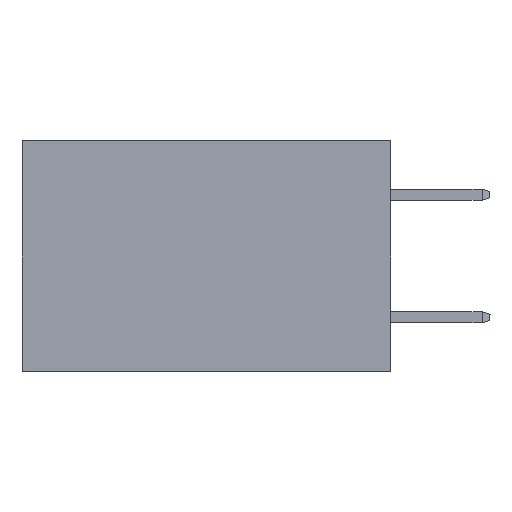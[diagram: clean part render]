
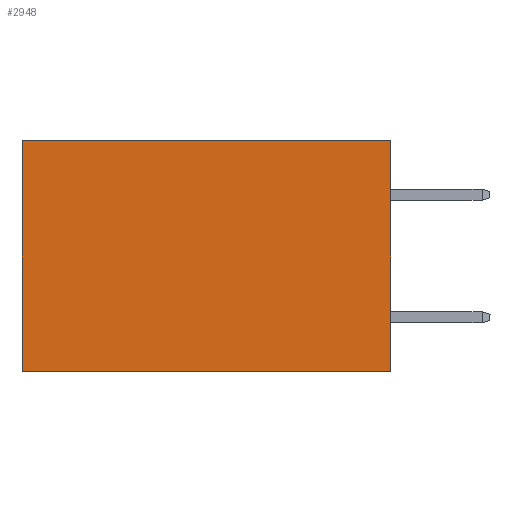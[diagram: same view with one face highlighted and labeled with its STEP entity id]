
A CAD part, left-side view. The second image highlights one B-rep face of the part: STEP entity #2948.
In plain terms, the highlighted planar face has unit normal (-1, 0, 0).
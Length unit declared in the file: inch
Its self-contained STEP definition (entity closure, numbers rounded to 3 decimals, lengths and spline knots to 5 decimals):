
#64 = VECTOR ( 'NONE', #7813, 39.37008 ) ;
#288 = EDGE_CURVE ( 'NONE', #19003, #20063, #1171, .T. ) ;
#1171 = LINE ( 'NONE', #4264, #17939 ) ;
#1609 = EDGE_CURVE ( 'NONE', #4205, #16646, #14479, .T. ) ;
#1852 = CARTESIAN_POINT ( 'NONE',  ( 0.2875, 0., -0.375 ) ) ;
#2948 = ADVANCED_FACE ( 'NONE', ( #13081 ), #15580, .F. ) ;
#3361 = LINE ( 'NONE', #10375, #5211 ) ;
#4205 = VERTEX_POINT ( 'NONE', #5260 ) ;
#4264 = CARTESIAN_POINT ( 'NONE',  ( 0.2875, 0., -0.375 ) ) ;
#5211 = VECTOR ( 'NONE', #13951, 39.37008 ) ;
#5260 = CARTESIAN_POINT ( 'NONE',  ( 0.2875, 0.6, 0. ) ) ;
#5610 = DIRECTION ( 'NONE',  ( 1., 0., 0. ) ) ;
#5905 = EDGE_LOOP ( 'NONE', ( #7347, #13079, #7869, #15262 ) ) ;
#7347 = ORIENTED_EDGE ( 'NONE', *, *, #1609, .T. ) ;
#7813 = DIRECTION ( 'NONE',  ( 0., 0., -1. ) ) ;
#7869 = ORIENTED_EDGE ( 'NONE', *, *, #288, .F. ) ;
#8055 = EDGE_CURVE ( 'NONE', #19003, #4205, #3361, .T. ) ;
#9043 = CARTESIAN_POINT ( 'NONE',  ( 0.2875, 0., -0.375 ) ) ;
#10295 = CARTESIAN_POINT ( 'NONE',  ( 0.2875, 0., -0.375 ) ) ;
#10375 = CARTESIAN_POINT ( 'NONE',  ( 0.2875, 0., 0. ) ) ;
#12633 = AXIS2_PLACEMENT_3D ( 'NONE', #9043, #5610, #15874 ) ;
#12679 = VECTOR ( 'NONE', #18633, 39.37008 ) ;
#13079 = ORIENTED_EDGE ( 'NONE', *, *, #14513, .F. ) ;
#13081 = FACE_OUTER_BOUND ( 'NONE', #5905, .T. ) ;
#13951 = DIRECTION ( 'NONE',  ( 0., 1., 0. ) ) ;
#14454 = CARTESIAN_POINT ( 'NONE',  ( 0.2875, 0.6, -0.375 ) ) ;
#14479 = LINE ( 'NONE', #14454, #64 ) ;
#14513 = EDGE_CURVE ( 'NONE', #20063, #16646, #21075, .T. ) ;
#15262 = ORIENTED_EDGE ( 'NONE', *, *, #8055, .T. ) ;
#15580 = PLANE ( 'NONE',  #12633 ) ;
#15804 = CARTESIAN_POINT ( 'NONE',  ( 0.2875, 0.6, -0.375 ) ) ;
#15874 = DIRECTION ( 'NONE',  ( 0., 0., -1. ) ) ;
#15881 = DIRECTION ( 'NONE',  ( 0., 0., -1. ) ) ;
#16646 = VERTEX_POINT ( 'NONE', #15804 ) ;
#17939 = VECTOR ( 'NONE', #15881, 39.37008 ) ;
#18633 = DIRECTION ( 'NONE',  ( 0., 1., 0. ) ) ;
#19003 = VERTEX_POINT ( 'NONE', #19539 ) ;
#19539 = CARTESIAN_POINT ( 'NONE',  ( 0.2875, 0., 0. ) ) ;
#20063 = VERTEX_POINT ( 'NONE', #10295 ) ;
#21075 = LINE ( 'NONE', #1852, #12679 ) ;
